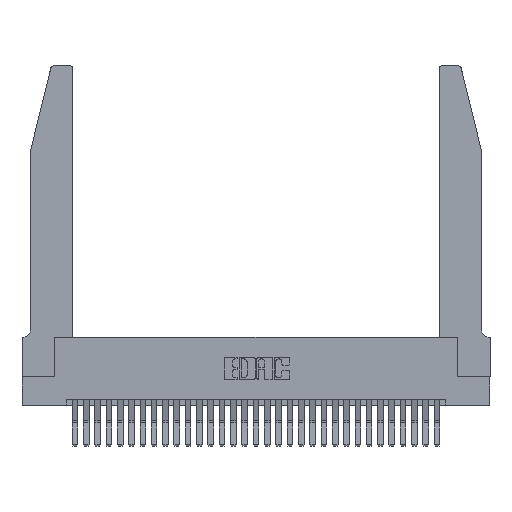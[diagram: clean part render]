
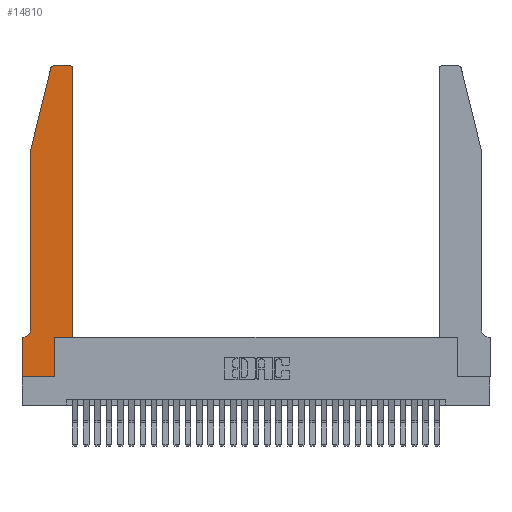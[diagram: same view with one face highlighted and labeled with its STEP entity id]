
A CAD part, top view. The second image highlights one B-rep face of the part: STEP entity #14810.
In plain terms, the highlighted planar face has unit normal (0, 0, 1).
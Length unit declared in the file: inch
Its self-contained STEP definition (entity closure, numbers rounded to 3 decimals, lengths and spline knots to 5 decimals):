
#54 = VERTEX_POINT ( 'NONE', #20341 ) ;
#82 = VERTEX_POINT ( 'NONE', #1104 ) ;
#226 = VERTEX_POINT ( 'NONE', #31230 ) ;
#393 = VECTOR ( 'NONE', #3179, 39.37008 ) ;
#546 = CARTESIAN_POINT ( 'NONE',  ( 0., 0., 0.37 ) ) ;
#988 = LINE ( 'NONE', #19731, #12922 ) ;
#1104 = CARTESIAN_POINT ( 'NONE',  ( 0., 0.35, 0.37 ) ) ;
#1671 = EDGE_CURVE ( 'NONE', #226, #7233, #11759, .T. ) ;
#1707 = CARTESIAN_POINT ( 'NONE',  ( 0.4505, 0.35, 0.37 ) ) ;
#1772 = DIRECTION ( 'NONE',  ( -1., 0., 0. ) ) ;
#2015 = DIRECTION ( 'NONE',  ( 1., 0., 0. ) ) ;
#2319 = CARTESIAN_POINT ( 'NONE',  ( 0.2865, 0., 0.37 ) ) ;
#3179 = DIRECTION ( 'NONE',  ( 1., 0., 0. ) ) ;
#3491 = VERTEX_POINT ( 'NONE', #21021 ) ;
#3971 = CARTESIAN_POINT ( 'NONE',  ( 0.2865, 0.35, 0.37 ) ) ;
#4264 = CARTESIAN_POINT ( 'NONE',  ( 0.0755, 0.42, 0.37 ) ) ;
#4303 = ORIENTED_EDGE ( 'NONE', *, *, #31179, .T. ) ;
#4518 = EDGE_CURVE ( 'NONE', #3491, #226, #6033, .T. ) ;
#4574 = EDGE_CURVE ( 'NONE', #82, #21036, #988, .T. ) ;
#4726 = PLANE ( 'NONE',  #25936 ) ;
#5044 = AXIS2_PLACEMENT_3D ( 'NONE', #31126, #8874, #1772 ) ;
#5977 = DIRECTION ( 'NONE',  ( 0., 0., 1. ) ) ;
#6033 = LINE ( 'NONE', #25647, #7538 ) ;
#6176 = DIRECTION ( 'NONE',  ( 0., 0., 1. ) ) ;
#7233 = VERTEX_POINT ( 'NONE', #4264 ) ;
#7405 = EDGE_CURVE ( 'NONE', #21036, #29195, #17031, .T. ) ;
#7535 = CARTESIAN_POINT ( 'NONE',  ( 0.0755, 0.35, 0.37 ) ) ;
#7538 = VECTOR ( 'NONE', #16594, 39.37008 ) ;
#7837 = FACE_OUTER_BOUND ( 'NONE', #9164, .T. ) ;
#7933 = LINE ( 'NONE', #30040, #19214 ) ;
#7940 = CIRCLE ( 'NONE', #31840, 0.03 ) ;
#8401 = DIRECTION ( 'NONE',  ( 1., 0., 0. ) ) ;
#8874 = DIRECTION ( 'NONE',  ( 0., 0., -1. ) ) ;
#9151 = VECTOR ( 'NONE', #10754, 39.37008 ) ;
#9164 = EDGE_LOOP ( 'NONE', ( #20839, #16396, #22792, #24673, #27630, #29407, #9498, #9553, #26308, #25273, #4303, #10778 ) ) ;
#9180 = DIRECTION ( 'NONE',  ( 1., 0., 0. ) ) ;
#9270 = VERTEX_POINT ( 'NONE', #1707 ) ;
#9477 = LINE ( 'NONE', #24194, #30735 ) ;
#9498 = ORIENTED_EDGE ( 'NONE', *, *, #4574, .T. ) ;
#9553 = ORIENTED_EDGE ( 'NONE', *, *, #7405, .T. ) ;
#9945 = CARTESIAN_POINT ( 'NONE',  ( 0.284, 2.75, 0.37 ) ) ;
#10754 = DIRECTION ( 'NONE',  ( -1., 0., 0. ) ) ;
#10778 = ORIENTED_EDGE ( 'NONE', *, *, #21079, .T. ) ;
#10961 = VERTEX_POINT ( 'NONE', #9945 ) ;
#11199 = VECTOR ( 'NONE', #13492, 39.37008 ) ;
#11590 = CARTESIAN_POINT ( 'NONE',  ( 0., 0.35, 0.37 ) ) ;
#11759 = LINE ( 'NONE', #15858, #25683 ) ;
#12922 = VECTOR ( 'NONE', #29753, 39.37008 ) ;
#13492 = DIRECTION ( 'NONE',  ( 0., 1., 0. ) ) ;
#13548 = CARTESIAN_POINT ( 'NONE',  ( 0.284, 2.72, 0.37 ) ) ;
#13561 = CARTESIAN_POINT ( 'NONE',  ( 0.4205, 2.75, 0.37 ) ) ;
#14401 = DIRECTION ( 'NONE',  ( 0., 0., 1. ) ) ;
#14810 = ADVANCED_FACE ( 'NONE', ( #7837 ), #4726, .T. ) ;
#15230 = DIRECTION ( 'NONE',  ( 0., 1., 0. ) ) ;
#15435 = CARTESIAN_POINT ( 'NONE',  ( 0., 0., 0.37 ) ) ;
#15723 = DIRECTION ( 'NONE',  ( 0., -1., 0. ) ) ;
#15858 = CARTESIAN_POINT ( 'NONE',  ( 0.0755, 2., 0.37 ) ) ;
#16396 = ORIENTED_EDGE ( 'NONE', *, *, #25833, .T. ) ;
#16594 = DIRECTION ( 'NONE',  ( -0.239, -0.971, 0. ) ) ;
#16680 = EDGE_CURVE ( 'NONE', #29413, #10961, #23943, .T. ) ;
#16781 = CARTESIAN_POINT ( 'NONE',  ( 0.0055, 0.35, 0.37 ) ) ;
#17031 = LINE ( 'NONE', #546, #393 ) ;
#17304 = VERTEX_POINT ( 'NONE', #16781 ) ;
#18288 = CARTESIAN_POINT ( 'NONE',  ( 0.4205, 2.72, 0.37 ) ) ;
#18756 = EDGE_CURVE ( 'NONE', #29195, #54, #22383, .T. ) ;
#19214 = VECTOR ( 'NONE', #15230, 39.37008 ) ;
#19731 = CARTESIAN_POINT ( 'NONE',  ( 0., 0., 0.37 ) ) ;
#20341 = CARTESIAN_POINT ( 'NONE',  ( 0.2865, 0.35, 0.37 ) ) ;
#20512 = CIRCLE ( 'NONE', #24275, 0.03 ) ;
#20839 = ORIENTED_EDGE ( 'NONE', *, *, #16680, .T. ) ;
#21021 = CARTESIAN_POINT ( 'NONE',  ( 0.25487, 2.72718, 0.37 ) ) ;
#21036 = VERTEX_POINT ( 'NONE', #15435 ) ;
#21079 = EDGE_CURVE ( 'NONE', #28620, #29413, #7940, .T. ) ;
#22383 = LINE ( 'NONE', #3971, #11199 ) ;
#22792 = ORIENTED_EDGE ( 'NONE', *, *, #4518, .T. ) ;
#23222 = DIRECTION ( 'NONE',  ( 1., 0., 0. ) ) ;
#23619 = CIRCLE ( 'NONE', #5044, 0.07 ) ;
#23899 = EDGE_CURVE ( 'NONE', #17304, #82, #26908, .T. ) ;
#23943 = LINE ( 'NONE', #29193, #30914 ) ;
#24194 = CARTESIAN_POINT ( 'NONE',  ( 0.4505, 0.35, 0.37 ) ) ;
#24275 = AXIS2_PLACEMENT_3D ( 'NONE', #13548, #6176, #8401 ) ;
#24673 = ORIENTED_EDGE ( 'NONE', *, *, #1671, .T. ) ;
#24929 = CARTESIAN_POINT ( 'NONE',  ( 0.4505, 2.72, 0.37 ) ) ;
#25273 = ORIENTED_EDGE ( 'NONE', *, *, #31492, .T. ) ;
#25375 = EDGE_CURVE ( 'NONE', #7233, #17304, #23619, .T. ) ;
#25647 = CARTESIAN_POINT ( 'NONE',  ( 0.0755, 2., 0.37 ) ) ;
#25683 = VECTOR ( 'NONE', #15723, 39.37008 ) ;
#25833 = EDGE_CURVE ( 'NONE', #10961, #3491, #20512, .T. ) ;
#25936 = AXIS2_PLACEMENT_3D ( 'NONE', #11590, #14401, #2015 ) ;
#26308 = ORIENTED_EDGE ( 'NONE', *, *, #18756, .T. ) ;
#26908 = LINE ( 'NONE', #7535, #9151 ) ;
#27630 = ORIENTED_EDGE ( 'NONE', *, *, #25375, .T. ) ;
#28620 = VERTEX_POINT ( 'NONE', #24929 ) ;
#29193 = CARTESIAN_POINT ( 'NONE',  ( 0.2605, 2.75, 0.37 ) ) ;
#29195 = VERTEX_POINT ( 'NONE', #2319 ) ;
#29407 = ORIENTED_EDGE ( 'NONE', *, *, #23899, .T. ) ;
#29413 = VERTEX_POINT ( 'NONE', #13561 ) ;
#29753 = DIRECTION ( 'NONE',  ( 0., -1., 0. ) ) ;
#30040 = CARTESIAN_POINT ( 'NONE',  ( 0.4505, 0.35, 0.37 ) ) ;
#30735 = VECTOR ( 'NONE', #9180, 39.37008 ) ;
#30914 = VECTOR ( 'NONE', #31678, 39.37008 ) ;
#31126 = CARTESIAN_POINT ( 'NONE',  ( 0.0055, 0.42, 0.37 ) ) ;
#31179 = EDGE_CURVE ( 'NONE', #9270, #28620, #7933, .T. ) ;
#31230 = CARTESIAN_POINT ( 'NONE',  ( 0.0755, 2., 0.37 ) ) ;
#31492 = EDGE_CURVE ( 'NONE', #54, #9270, #9477, .T. ) ;
#31678 = DIRECTION ( 'NONE',  ( -1., 0., 0. ) ) ;
#31840 = AXIS2_PLACEMENT_3D ( 'NONE', #18288, #5977, #23222 ) ;
